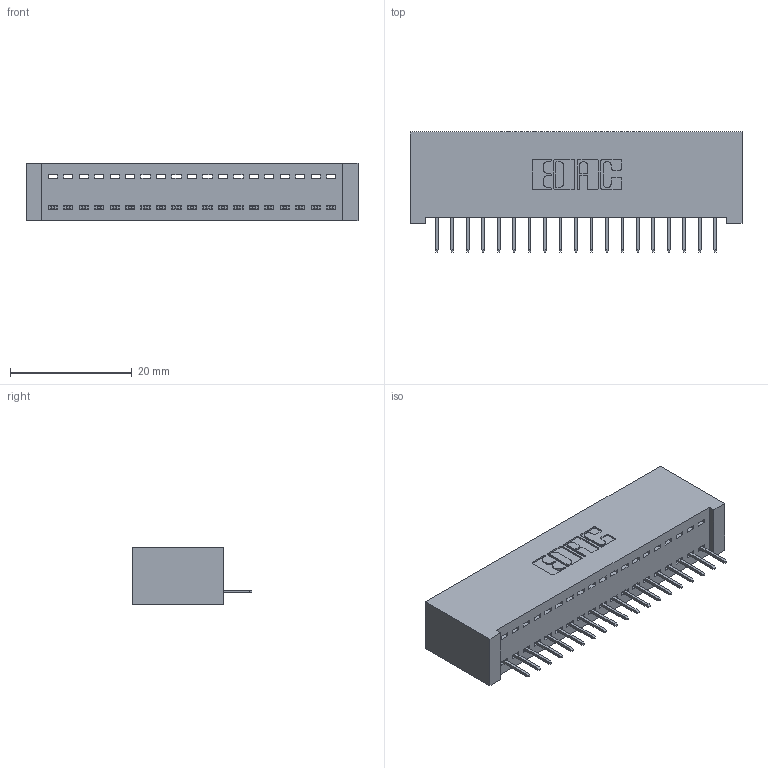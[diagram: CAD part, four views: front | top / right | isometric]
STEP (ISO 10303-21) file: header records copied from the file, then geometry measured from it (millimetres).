
FILE_DESCRIPTION (( 'STEP AP203' ), '1' );
FILE_NAME ('392-019-524-101.STEP', '2019-10-07T04:37:43', ( '' ), ( '' ), 'SwSTEP 2.0', 'SolidWorks 2016', '' );
FILE_SCHEMA (( 'CONFIG_CONTROL_DESIGN' ));
Length unit declared in the file: inch
Products named in the file (3): 392-019-524-101; 342 Part_Lugless; 345-292-001_345-293-124
Assembly tree (20 placements, depth 2):
  392-019-524-101
    342 Part_Lugless
    345-292-001_345-293-124  x19
Bounding box: 54.51 x 19.69 x 9.4 mm (x, y, z)
Volume: 5028.5 mm3; surface area: 7044.8 mm2
Topology: 20 solids, 20 shells, 1280 faces, 3695 edges, 2386 vertices
Faces by surface type: plane 974, cylinder 306
Entity records: 14255 total; most frequent: CARTESIAN_POINT 2467, ORIENTED_EDGE 2422, DIRECTION 2121, EDGE_CURVE 1211, LINE 1095, VECTOR 1095, VERTEX_POINT 802, AXIS2_PLACEMENT_3D 513
